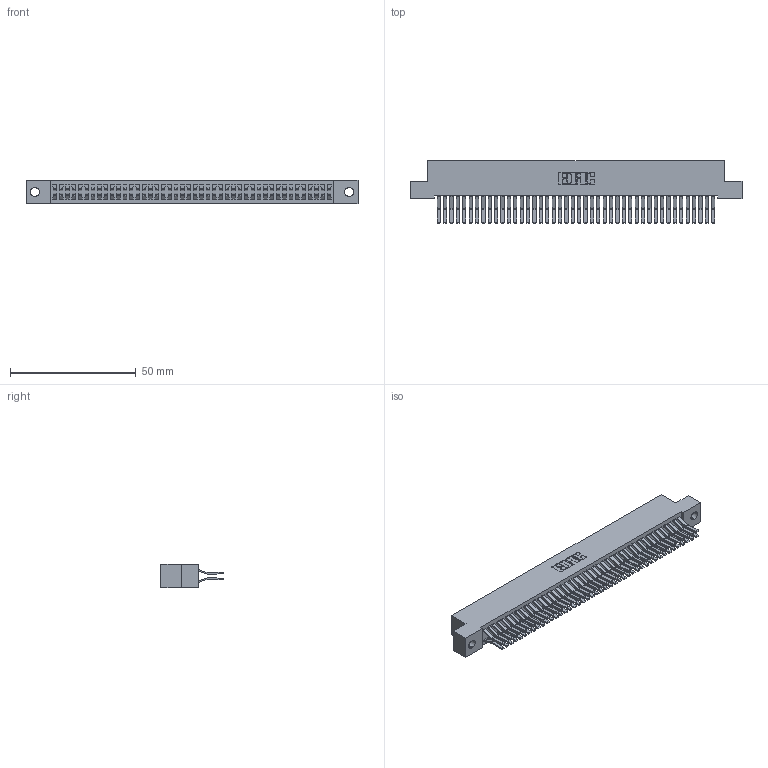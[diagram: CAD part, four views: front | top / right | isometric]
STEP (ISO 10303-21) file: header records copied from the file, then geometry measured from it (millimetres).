
FILE_DESCRIPTION (( 'STEP AP203' ), '1' );
FILE_NAME ('392-088-560-202.STEP', '2019-10-09T17:08:36', ( '' ), ( '' ), 'SwSTEP 2.0', 'SolidWorks 2016', '' );
FILE_SCHEMA (( 'CONFIG_CONTROL_DESIGN' ));
Length unit declared in the file: inch
Products named in the file (3): 345-292-001_560 Tail; 392-088-560-202; 342 Part_.128 Slot
Assembly tree (89 placements, depth 2):
  392-088-560-202
    342 Part_.128 Slot
    345-292-001_560 Tail  x88
Bounding box: 132.08 x 24.78 x 9.4 mm (x, y, z)
Volume: 12402.4 mm3; surface area: 21382.2 mm2
Topology: 89 solids, 89 shells, 4866 faces, 14479 edges, 9534 vertices
Faces by surface type: plane 3238, cylinder 1628
Entity records: 28139 total; most frequent: CARTESIAN_POINT 4662, ORIENTED_EDGE 4598, DIRECTION 3983, EDGE_CURVE 2299, VECTOR 2167, LINE 2167, VERTEX_POINT 1530, AXIS2_PLACEMENT_3D 908
